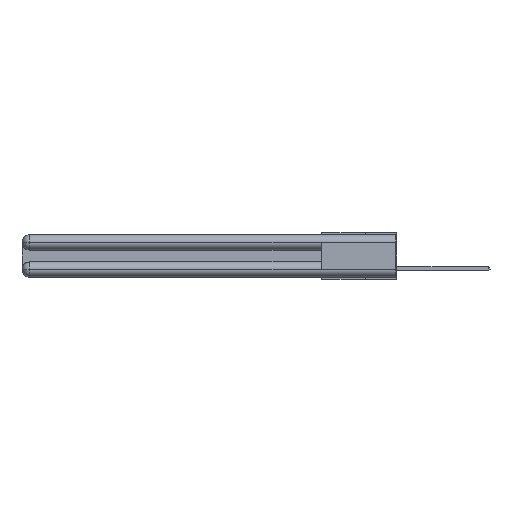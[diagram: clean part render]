
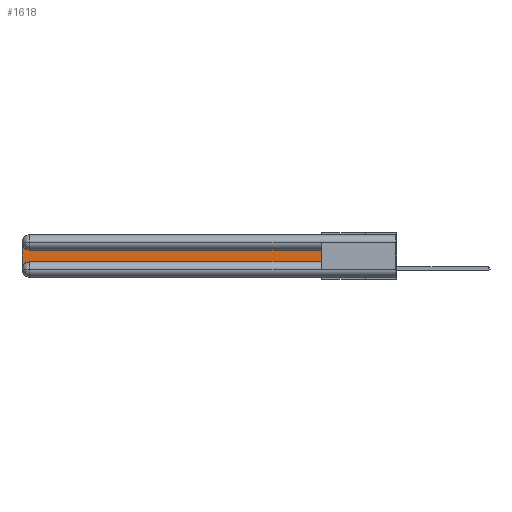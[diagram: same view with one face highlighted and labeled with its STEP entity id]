
A CAD part, left-side view. The second image highlights one B-rep face of the part: STEP entity #1618.
In plain terms, the highlighted planar face has unit normal (-1, 0, 0).
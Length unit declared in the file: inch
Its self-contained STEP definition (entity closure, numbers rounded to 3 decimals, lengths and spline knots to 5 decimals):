
#1618 = ADVANCED_FACE ( 'NONE', ( #16677 ), #4063, .F. ) ;
#3093 = VERTEX_POINT ( 'NONE', #28131 ) ;
#4063 = PLANE ( 'NONE',  #31710 ) ;
#4606 = VECTOR ( 'NONE', #16624, 39.37008 ) ;
#4727 = ORIENTED_EDGE ( 'NONE', *, *, #25302, .T. ) ;
#4782 = DIRECTION ( 'NONE',  ( 1., 0., 0. ) ) ;
#5317 = ORIENTED_EDGE ( 'NONE', *, *, #6374, .T. ) ;
#5745 = DIRECTION ( 'NONE',  ( 0., 0., -1. ) ) ;
#6374 = EDGE_CURVE ( 'NONE', #28084, #31814, #16514, .T. ) ;
#7055 = VERTEX_POINT ( 'NONE', #8396 ) ;
#7599 = AXIS2_PLACEMENT_3D ( 'NONE', #21571, #9091, #26599 ) ;
#7867 = VERTEX_POINT ( 'NONE', #23860 ) ;
#8396 = CARTESIAN_POINT ( 'NONE',  ( 0.075, 2.94, -0.1225 ) ) ;
#8676 = DIRECTION ( 'NONE',  ( 0., 1., 0. ) ) ;
#9091 = DIRECTION ( 'NONE',  ( 1., 0., 0. ) ) ;
#13440 = AXIS2_PLACEMENT_3D ( 'NONE', #27537, #4782, #20186 ) ;
#14142 = VECTOR ( 'NONE', #5745, 39.37008 ) ;
#15846 = EDGE_CURVE ( 'NONE', #7055, #28084, #27144, .T. ) ;
#16057 = ORIENTED_EDGE ( 'NONE', *, *, #15846, .T. ) ;
#16514 = LINE ( 'NONE', #30490, #14142 ) ;
#16624 = DIRECTION ( 'NONE',  ( 0., 0., 1. ) ) ;
#16677 = FACE_OUTER_BOUND ( 'NONE', #30349, .T. ) ;
#17109 = LINE ( 'NONE', #24032, #4606 ) ;
#17389 = CARTESIAN_POINT ( 'NONE',  ( 0.075, 0.6, -0.1225 ) ) ;
#18245 = ORIENTED_EDGE ( 'NONE', *, *, #24736, .T. ) ;
#18871 = VECTOR ( 'NONE', #28856, 39.37008 ) ;
#18939 = DIRECTION ( 'NONE',  ( 1., 0., 0. ) ) ;
#19987 = ORIENTED_EDGE ( 'NONE', *, *, #29976, .T. ) ;
#20186 = DIRECTION ( 'NONE',  ( 0., 0., -1. ) ) ;
#21213 = CARTESIAN_POINT ( 'NONE',  ( 0.075, 3., -0.1225 ) ) ;
#21571 = CARTESIAN_POINT ( 'NONE',  ( 0.075, 2.94, -0.2775 ) ) ;
#23860 = CARTESIAN_POINT ( 'NONE',  ( 0.075, 2.94, -0.2175 ) ) ;
#24032 = CARTESIAN_POINT ( 'NONE',  ( 0.075, 0.6, -0.2175 ) ) ;
#24736 = EDGE_CURVE ( 'NONE', #7867, #3093, #31830, .T. ) ;
#24885 = CIRCLE ( 'NONE', #7599, 0.06 ) ;
#25093 = ORIENTED_EDGE ( 'NONE', *, *, #27026, .T. ) ;
#25302 = EDGE_CURVE ( 'NONE', #26707, #7055, #30610, .T. ) ;
#26586 = DIRECTION ( 'NONE',  ( 0., 0., -1. ) ) ;
#26599 = DIRECTION ( 'NONE',  ( 0., 0., -1. ) ) ;
#26707 = VERTEX_POINT ( 'NONE', #17389 ) ;
#27026 = EDGE_CURVE ( 'NONE', #3093, #26707, #17109, .T. ) ;
#27144 = CIRCLE ( 'NONE', #13440, 0.06 ) ;
#27537 = CARTESIAN_POINT ( 'NONE',  ( 0.075, 2.94, -0.0625 ) ) ;
#28084 = VERTEX_POINT ( 'NONE', #29840 ) ;
#28131 = CARTESIAN_POINT ( 'NONE',  ( 0.075, 0.6, -0.2175 ) ) ;
#28703 = CARTESIAN_POINT ( 'NONE',  ( 0.075, 0.6, -0.1225 ) ) ;
#28856 = DIRECTION ( 'NONE',  ( 0., -1., 0. ) ) ;
#29197 = CARTESIAN_POINT ( 'NONE',  ( 0.075, 0.6, -0.2175 ) ) ;
#29592 = CARTESIAN_POINT ( 'NONE',  ( 0.075, 3., -0.2775 ) ) ;
#29840 = CARTESIAN_POINT ( 'NONE',  ( 0.075, 3., -0.0625 ) ) ;
#29976 = EDGE_CURVE ( 'NONE', #31814, #7867, #24885, .T. ) ;
#30349 = EDGE_LOOP ( 'NONE', ( #4727, #16057, #5317, #19987, #18245, #25093 ) ) ;
#30490 = CARTESIAN_POINT ( 'NONE',  ( 0.075, 3., -0.2175 ) ) ;
#30610 = LINE ( 'NONE', #28703, #31769 ) ;
#31710 = AXIS2_PLACEMENT_3D ( 'NONE', #21213, #18939, #26586 ) ;
#31769 = VECTOR ( 'NONE', #8676, 39.37008 ) ;
#31814 = VERTEX_POINT ( 'NONE', #29592 ) ;
#31830 = LINE ( 'NONE', #29197, #18871 ) ;
